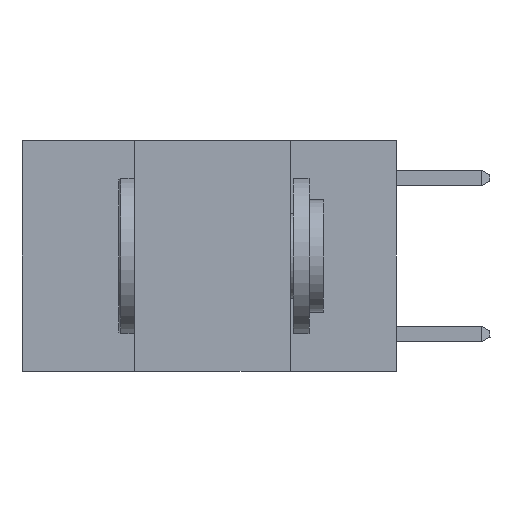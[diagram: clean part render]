
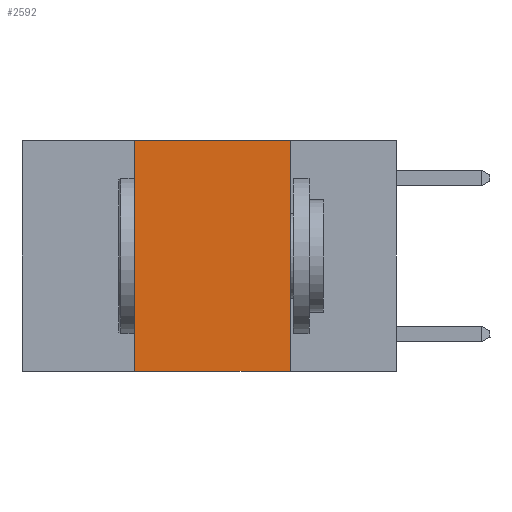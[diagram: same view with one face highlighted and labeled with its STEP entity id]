
A CAD part, left-side view. The second image highlights one B-rep face of the part: STEP entity #2592.
In plain terms, the highlighted planar face has unit normal (-1, 0, 0).
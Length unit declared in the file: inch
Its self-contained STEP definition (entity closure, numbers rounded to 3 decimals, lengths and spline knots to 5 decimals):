
#69 = PLANE ( 'NONE',  #10157 ) ;
#412 = EDGE_CURVE ( 'NONE', #9522, #2752, #8277, .T. ) ;
#2397 = FACE_OUTER_BOUND ( 'NONE', #11246, .T. ) ;
#2592 = ADVANCED_FACE ( 'NONE', ( #2397 ), #69, .F. ) ;
#2752 = VERTEX_POINT ( 'NONE', #4454 ) ;
#3972 = DIRECTION ( 'NONE',  ( 0., 0., -1. ) ) ;
#4410 = VERTEX_POINT ( 'NONE', #19197 ) ;
#4454 = CARTESIAN_POINT ( 'NONE',  ( 0., 0.17, 0. ) ) ;
#4667 = LINE ( 'NONE', #13927, #13834 ) ;
#6576 = EDGE_CURVE ( 'NONE', #4410, #9522, #18197, .T. ) ;
#6677 = ORIENTED_EDGE ( 'NONE', *, *, #12707, .F. ) ;
#6754 = ORIENTED_EDGE ( 'NONE', *, *, #412, .F. ) ;
#6804 = ORIENTED_EDGE ( 'NONE', *, *, #6576, .F. ) ;
#7256 = ORIENTED_EDGE ( 'NONE', *, *, #7849, .T. ) ;
#7849 = EDGE_CURVE ( 'NONE', #4410, #15802, #11726, .T. ) ;
#8086 = VECTOR ( 'NONE', #14782, 39.37008 ) ;
#8277 = LINE ( 'NONE', #12760, #8086 ) ;
#8345 = DIRECTION ( 'NONE',  ( 0., 0., 1. ) ) ;
#9522 = VERTEX_POINT ( 'NONE', #19815 ) ;
#10157 = AXIS2_PLACEMENT_3D ( 'NONE', #13112, #14975, #3972 ) ;
#10192 = DIRECTION ( 'NONE',  ( 0., -1., 0. ) ) ;
#11246 = EDGE_LOOP ( 'NONE', ( #6677, #6754, #6804, #7256 ) ) ;
#11382 = CARTESIAN_POINT ( 'NONE',  ( 0., 0.17, -0.37 ) ) ;
#11726 = LINE ( 'NONE', #15712, #11831 ) ;
#11831 = VECTOR ( 'NONE', #10192, 39.37008 ) ;
#12707 = EDGE_CURVE ( 'NONE', #2752, #15802, #4667, .T. ) ;
#12760 = CARTESIAN_POINT ( 'NONE',  ( 0., 0.6, 0. ) ) ;
#13112 = CARTESIAN_POINT ( 'NONE',  ( 0., 0.6, 0. ) ) ;
#13834 = VECTOR ( 'NONE', #21125, 39.37008 ) ;
#13927 = CARTESIAN_POINT ( 'NONE',  ( 0., 0.17, 0. ) ) ;
#14782 = DIRECTION ( 'NONE',  ( 0., -1., 0. ) ) ;
#14975 = DIRECTION ( 'NONE',  ( 1., 0., 0. ) ) ;
#15712 = CARTESIAN_POINT ( 'NONE',  ( 0., 0.6, -0.37 ) ) ;
#15802 = VERTEX_POINT ( 'NONE', #11382 ) ;
#17954 = VECTOR ( 'NONE', #8345, 39.37008 ) ;
#18197 = LINE ( 'NONE', #20981, #17954 ) ;
#19197 = CARTESIAN_POINT ( 'NONE',  ( 0., 0.42, -0.37 ) ) ;
#19815 = CARTESIAN_POINT ( 'NONE',  ( 0., 0.42, 0. ) ) ;
#20981 = CARTESIAN_POINT ( 'NONE',  ( 0., 0.42, 0. ) ) ;
#21125 = DIRECTION ( 'NONE',  ( 0., 0., -1. ) ) ;
